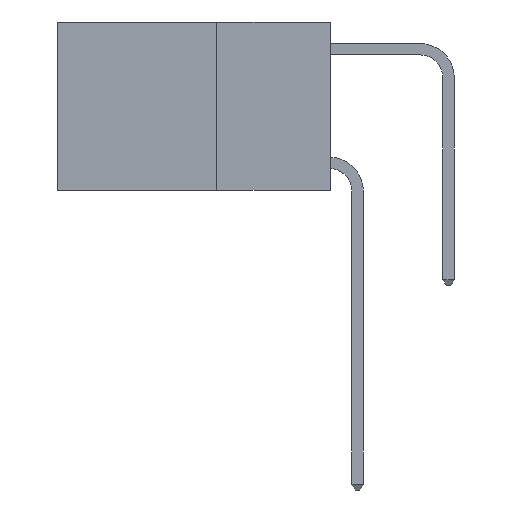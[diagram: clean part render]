
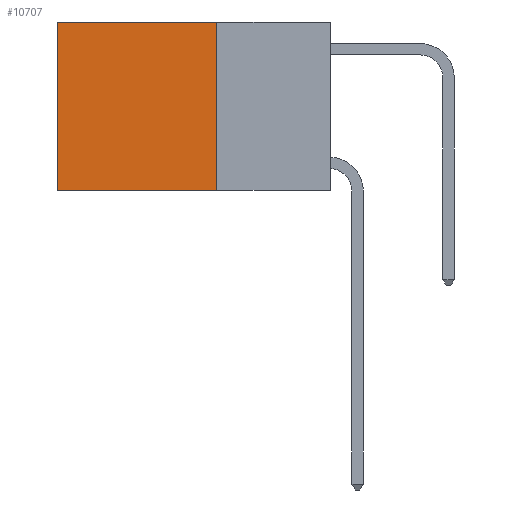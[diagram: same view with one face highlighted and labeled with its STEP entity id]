
A CAD part, left-side view. The second image highlights one B-rep face of the part: STEP entity #10707.
In plain terms, the highlighted planar face has unit normal (-1, 0, 0).
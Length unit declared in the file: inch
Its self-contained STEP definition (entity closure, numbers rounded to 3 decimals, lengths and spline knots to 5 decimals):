
#289 = CARTESIAN_POINT ( 'NONE',  ( 0.2625, 0.6, 0. ) ) ;
#456 = EDGE_CURVE ( 'NONE', #562, #6761, #9343, .T. ) ;
#562 = VERTEX_POINT ( 'NONE', #289 ) ;
#788 = VECTOR ( 'NONE', #5326, 39.37008 ) ;
#1058 = VERTEX_POINT ( 'NONE', #1277 ) ;
#1277 = CARTESIAN_POINT ( 'NONE',  ( 0.2625, 0.25, -0.37 ) ) ;
#2114 = VECTOR ( 'NONE', #3869, 39.37008 ) ;
#2242 = DIRECTION ( 'NONE',  ( 0., 0., -1. ) ) ;
#2766 = VECTOR ( 'NONE', #2242, 39.37008 ) ;
#3869 = DIRECTION ( 'NONE',  ( 0., 1., 0. ) ) ;
#4444 = ORIENTED_EDGE ( 'NONE', *, *, #11450, .T. ) ;
#4903 = CARTESIAN_POINT ( 'NONE',  ( 0.2625, 0.25, -0.37 ) ) ;
#5267 = VECTOR ( 'NONE', #10001, 39.37008 ) ;
#5326 = DIRECTION ( 'NONE',  ( 0., 1., 0. ) ) ;
#5494 = ORIENTED_EDGE ( 'NONE', *, *, #456, .T. ) ;
#5504 = EDGE_CURVE ( 'NONE', #11525, #1058, #8408, .T. ) ;
#5523 = DIRECTION ( 'NONE',  ( 1., 0., 0. ) ) ;
#5823 = CARTESIAN_POINT ( 'NONE',  ( 0.2625, 0.25, 0. ) ) ;
#6761 = VERTEX_POINT ( 'NONE', #7880 ) ;
#6957 = ORIENTED_EDGE ( 'NONE', *, *, #5504, .F. ) ;
#7462 = CARTESIAN_POINT ( 'NONE',  ( 0.2625, 0.25, 0. ) ) ;
#7554 = CARTESIAN_POINT ( 'NONE',  ( 0.2625, 0.25, 0. ) ) ;
#7880 = CARTESIAN_POINT ( 'NONE',  ( 0.2625, 0.6, -0.37 ) ) ;
#8252 = EDGE_LOOP ( 'NONE', ( #5494, #9085, #6957, #4444 ) ) ;
#8408 = LINE ( 'NONE', #5823, #5267 ) ;
#8670 = CARTESIAN_POINT ( 'NONE',  ( 0.2625, 0.25, 0. ) ) ;
#9085 = ORIENTED_EDGE ( 'NONE', *, *, #11803, .F. ) ;
#9343 = LINE ( 'NONE', #12631, #2766 ) ;
#10001 = DIRECTION ( 'NONE',  ( 0., 0., -1. ) ) ;
#10224 = AXIS2_PLACEMENT_3D ( 'NONE', #8670, #5523, #12781 ) ;
#10496 = LINE ( 'NONE', #4903, #2114 ) ;
#10707 = ADVANCED_FACE ( 'NONE', ( #12436 ), #11751, .F. ) ;
#11450 = EDGE_CURVE ( 'NONE', #11525, #562, #11930, .T. ) ;
#11525 = VERTEX_POINT ( 'NONE', #7554 ) ;
#11751 = PLANE ( 'NONE',  #10224 ) ;
#11803 = EDGE_CURVE ( 'NONE', #1058, #6761, #10496, .T. ) ;
#11930 = LINE ( 'NONE', #7462, #788 ) ;
#12436 = FACE_OUTER_BOUND ( 'NONE', #8252, .T. ) ;
#12631 = CARTESIAN_POINT ( 'NONE',  ( 0.2625, 0.6, 0. ) ) ;
#12781 = DIRECTION ( 'NONE',  ( 0., 0., -1. ) ) ;
